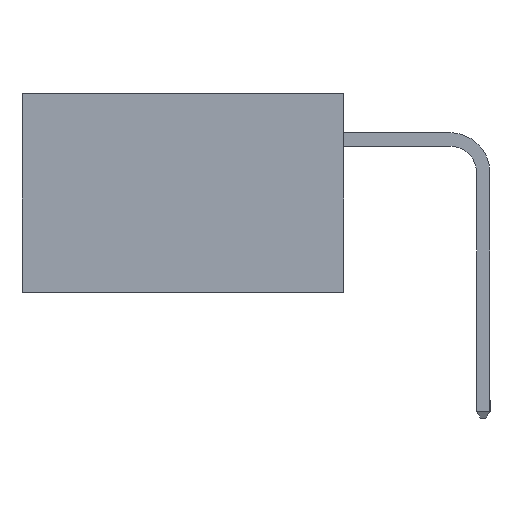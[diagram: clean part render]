
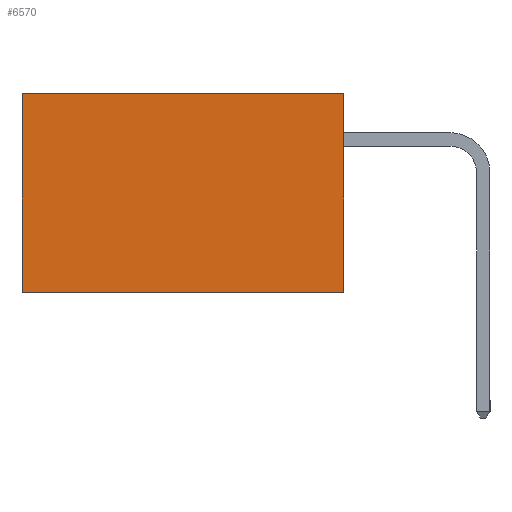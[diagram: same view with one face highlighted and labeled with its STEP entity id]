
A CAD part, left-side view. The second image highlights one B-rep face of the part: STEP entity #6570.
In plain terms, the highlighted planar face has unit normal (-1, 0, 0).
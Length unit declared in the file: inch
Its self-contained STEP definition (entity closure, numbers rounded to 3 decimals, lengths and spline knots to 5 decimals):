
#842 = CARTESIAN_POINT ( 'NONE',  ( 0.2615, 0.6, -0.37 ) ) ;
#1007 = FACE_OUTER_BOUND ( 'NONE', #9971, .T. ) ;
#2061 = ORIENTED_EDGE ( 'NONE', *, *, #11891, .F. ) ;
#2524 = CARTESIAN_POINT ( 'NONE',  ( 0.2615, 0., 0. ) ) ;
#3150 = EDGE_CURVE ( 'NONE', #24585, #6796, #22365, .T. ) ;
#3437 = CARTESIAN_POINT ( 'NONE',  ( 0.2615, 0.6, -0.37 ) ) ;
#3500 = ORIENTED_EDGE ( 'NONE', *, *, #13083, .F. ) ;
#3714 = VERTEX_POINT ( 'NONE', #16198 ) ;
#4882 = LINE ( 'NONE', #12855, #19904 ) ;
#5096 = LINE ( 'NONE', #19914, #14972 ) ;
#6570 = ADVANCED_FACE ( 'NONE', ( #1007 ), #11933, .F. ) ;
#6796 = VERTEX_POINT ( 'NONE', #23632 ) ;
#9338 = DIRECTION ( 'NONE',  ( 0., 0., -1. ) ) ;
#9971 = EDGE_LOOP ( 'NONE', ( #20251, #3500, #2061, #14064 ) ) ;
#11788 = DIRECTION ( 'NONE',  ( 0., 0., -1. ) ) ;
#11820 = DIRECTION ( 'NONE',  ( 1., 0., 0. ) ) ;
#11891 = EDGE_CURVE ( 'NONE', #24585, #3714, #4882, .T. ) ;
#11933 = PLANE ( 'NONE',  #12313 ) ;
#12313 = AXIS2_PLACEMENT_3D ( 'NONE', #12775, #11820, #11788 ) ;
#12775 = CARTESIAN_POINT ( 'NONE',  ( 0.2615, 0., -0.37 ) ) ;
#12855 = CARTESIAN_POINT ( 'NONE',  ( 0.2615, 0., -0.37 ) ) ;
#13083 = EDGE_CURVE ( 'NONE', #3714, #14481, #5096, .T. ) ;
#14064 = ORIENTED_EDGE ( 'NONE', *, *, #3150, .T. ) ;
#14481 = VERTEX_POINT ( 'NONE', #842 ) ;
#14835 = VECTOR ( 'NONE', #9338, 39.37008 ) ;
#14972 = VECTOR ( 'NONE', #21858, 39.37008 ) ;
#16198 = CARTESIAN_POINT ( 'NONE',  ( 0.2615, 0., -0.37 ) ) ;
#16233 = EDGE_CURVE ( 'NONE', #6796, #14481, #25086, .T. ) ;
#17213 = VECTOR ( 'NONE', #23152, 39.37008 ) ;
#18650 = DIRECTION ( 'NONE',  ( 0., 0., -1. ) ) ;
#19904 = VECTOR ( 'NONE', #18650, 39.37008 ) ;
#19914 = CARTESIAN_POINT ( 'NONE',  ( 0.2615, 0., -0.37 ) ) ;
#20251 = ORIENTED_EDGE ( 'NONE', *, *, #16233, .T. ) ;
#21858 = DIRECTION ( 'NONE',  ( 0., 1., 0. ) ) ;
#22365 = LINE ( 'NONE', #23311, #17213 ) ;
#23152 = DIRECTION ( 'NONE',  ( 0., 1., 0. ) ) ;
#23311 = CARTESIAN_POINT ( 'NONE',  ( 0.2615, 0., 0. ) ) ;
#23632 = CARTESIAN_POINT ( 'NONE',  ( 0.2615, 0.6, 0. ) ) ;
#24585 = VERTEX_POINT ( 'NONE', #2524 ) ;
#25086 = LINE ( 'NONE', #3437, #14835 ) ;
